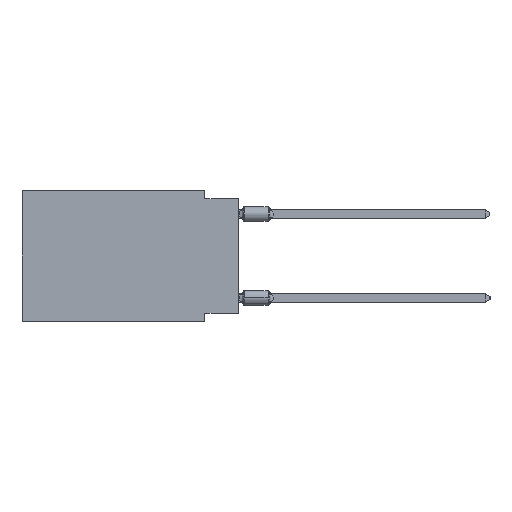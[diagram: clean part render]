
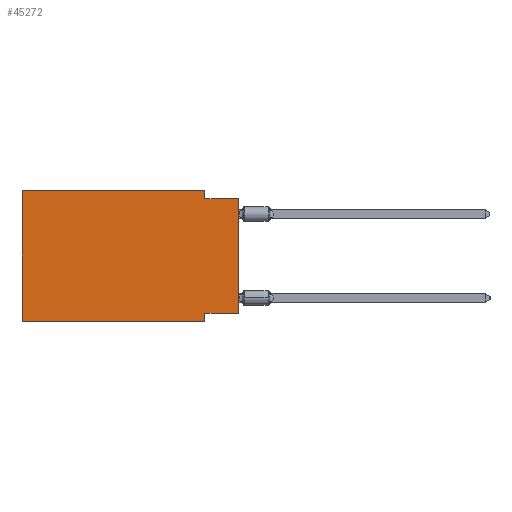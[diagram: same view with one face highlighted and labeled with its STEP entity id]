
A CAD part, left-side view. The second image highlights one B-rep face of the part: STEP entity #45272.
In plain terms, the highlighted planar face has unit normal (-1, 0, 0).
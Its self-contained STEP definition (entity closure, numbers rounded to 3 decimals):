
#1243 = ORIENTED_EDGE ( 'NONE', *, *, #58237, .F. ) ;
#1266 = ORIENTED_EDGE ( 'NONE', *, *, #14672, .F. ) ;
#3018 = LINE ( 'NONE', #35384, #34195 ) ;
#3387 = LINE ( 'NONE', #22267, #17261 ) ;
#7004 = VERTEX_POINT ( 'NONE', #58105 ) ;
#7101 = EDGE_CURVE ( 'NONE', #15283, #48179, #8385, .T. ) ;
#8385 = LINE ( 'NONE', #30853, #38946 ) ;
#8567 = PLANE ( 'NONE',  #31224 ) ;
#8706 = VECTOR ( 'NONE', #53821, 1000. ) ;
#9273 = VERTEX_POINT ( 'NONE', #32200 ) ;
#10883 = CARTESIAN_POINT ( 'NONE',  ( 0., 0., -0.635 ) ) ;
#14493 = CARTESIAN_POINT ( 'NONE',  ( 0., 16.383, 0. ) ) ;
#14604 = ORIENTED_EDGE ( 'NONE', *, *, #35499, .F. ) ;
#14615 = LINE ( 'NONE', #18218, #52619 ) ;
#14672 = EDGE_CURVE ( 'NONE', #45070, #15283, #17585, .T. ) ;
#15283 = VERTEX_POINT ( 'NONE', #14493 ) ;
#15397 = LINE ( 'NONE', #10883, #39678 ) ;
#16513 = CARTESIAN_POINT ( 'NONE',  ( 0., 2.54, 0. ) ) ;
#16894 = DIRECTION ( 'NONE',  ( 0., 0., -1. ) ) ;
#17261 = VECTOR ( 'NONE', #16894, 1000. ) ;
#17585 = LINE ( 'NONE', #43954, #8706 ) ;
#18218 = CARTESIAN_POINT ( 'NONE',  ( 0., 2.54, -9.906 ) ) ;
#19047 = CARTESIAN_POINT ( 'NONE',  ( 0., 16.383, 0. ) ) ;
#22267 = CARTESIAN_POINT ( 'NONE',  ( 0., 2.54, 0. ) ) ;
#22883 = DIRECTION ( 'NONE',  ( 0., -1., 0. ) ) ;
#23190 = EDGE_CURVE ( 'NONE', #45070, #23489, #40864, .T. ) ;
#23489 = VERTEX_POINT ( 'NONE', #38438 ) ;
#26114 = CARTESIAN_POINT ( 'NONE',  ( 0., 0., -0.635 ) ) ;
#26654 = VECTOR ( 'NONE', #22883, 1000. ) ;
#26985 = ORIENTED_EDGE ( 'NONE', *, *, #52565, .F. ) ;
#28411 = VERTEX_POINT ( 'NONE', #26114 ) ;
#30853 = CARTESIAN_POINT ( 'NONE',  ( 0., 16.383, 0. ) ) ;
#31049 = ORIENTED_EDGE ( 'NONE', *, *, #51927, .F. ) ;
#31224 = AXIS2_PLACEMENT_3D ( 'NONE', #19047, #36415, #49886 ) ;
#31977 = ORIENTED_EDGE ( 'NONE', *, *, #7101, .F. ) ;
#32200 = CARTESIAN_POINT ( 'NONE',  ( 0., 2.54, -0.635 ) ) ;
#33072 = DIRECTION ( 'NONE',  ( 0., -1., 0. ) ) ;
#34195 = VECTOR ( 'NONE', #48559, 1000. ) ;
#35289 = EDGE_CURVE ( 'NONE', #7004, #28411, #36328, .T. ) ;
#35384 = CARTESIAN_POINT ( 'NONE',  ( 0., 0., -9.271 ) ) ;
#35499 = EDGE_CURVE ( 'NONE', #7004, #35574, #3018, .T. ) ;
#35574 = VERTEX_POINT ( 'NONE', #45248 ) ;
#36122 = FACE_OUTER_BOUND ( 'NONE', #54973, .T. ) ;
#36328 = LINE ( 'NONE', #45321, #52365 ) ;
#36415 = DIRECTION ( 'NONE',  ( 1., 0., 0. ) ) ;
#37678 = DIRECTION ( 'NONE',  ( 0., 0., -1. ) ) ;
#38438 = CARTESIAN_POINT ( 'NONE',  ( 0., 2.54, -9.906 ) ) ;
#38946 = VECTOR ( 'NONE', #53912, 1000. ) ;
#39678 = VECTOR ( 'NONE', #33072, 1000. ) ;
#40864 = LINE ( 'NONE', #54627, #26654 ) ;
#43954 = CARTESIAN_POINT ( 'NONE',  ( 0., 16.383, 0. ) ) ;
#45070 = VERTEX_POINT ( 'NONE', #56533 ) ;
#45248 = CARTESIAN_POINT ( 'NONE',  ( 0., 2.54, -9.271 ) ) ;
#45272 = ADVANCED_FACE ( 'NONE', ( #36122 ), #8567, .F. ) ;
#45321 = CARTESIAN_POINT ( 'NONE',  ( 0., 0., 0. ) ) ;
#48179 = VERTEX_POINT ( 'NONE', #16513 ) ;
#48559 = DIRECTION ( 'NONE',  ( 0., 1., 0. ) ) ;
#49886 = DIRECTION ( 'NONE',  ( 0., 0., -1. ) ) ;
#51611 = ORIENTED_EDGE ( 'NONE', *, *, #35289, .T. ) ;
#51927 = EDGE_CURVE ( 'NONE', #35574, #23489, #14615, .T. ) ;
#52365 = VECTOR ( 'NONE', #55481, 1000. ) ;
#52565 = EDGE_CURVE ( 'NONE', #48179, #9273, #3387, .T. ) ;
#52619 = VECTOR ( 'NONE', #37678, 1000. ) ;
#52753 = ORIENTED_EDGE ( 'NONE', *, *, #23190, .T. ) ;
#53821 = DIRECTION ( 'NONE',  ( 0., 0., 1. ) ) ;
#53912 = DIRECTION ( 'NONE',  ( 0., -1., 0. ) ) ;
#54627 = CARTESIAN_POINT ( 'NONE',  ( 0., 16.383, -9.906 ) ) ;
#54973 = EDGE_LOOP ( 'NONE', ( #51611, #1243, #26985, #31977, #1266, #52753, #31049, #14604 ) ) ;
#55481 = DIRECTION ( 'NONE',  ( 0., 0., 1. ) ) ;
#56533 = CARTESIAN_POINT ( 'NONE',  ( 0., 16.383, -9.906 ) ) ;
#58105 = CARTESIAN_POINT ( 'NONE',  ( 0., 0., -9.271 ) ) ;
#58237 = EDGE_CURVE ( 'NONE', #9273, #28411, #15397, .T. ) ;
